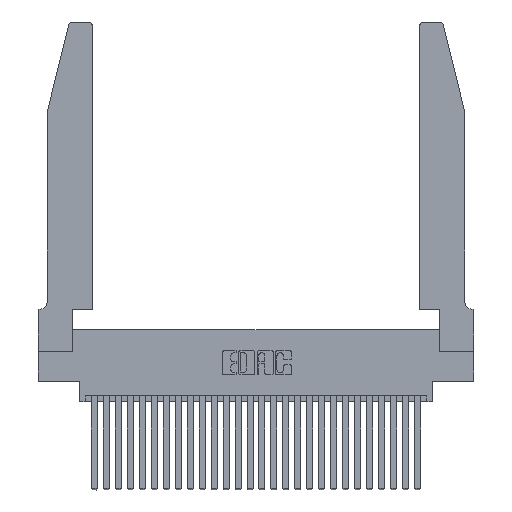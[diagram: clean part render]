
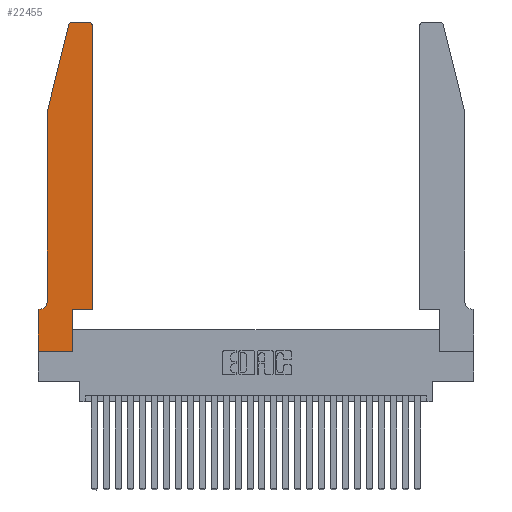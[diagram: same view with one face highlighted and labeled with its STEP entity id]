
A CAD part, top view. The second image highlights one B-rep face of the part: STEP entity #22455.
In plain terms, the highlighted planar face has unit normal (0, 0, 1).
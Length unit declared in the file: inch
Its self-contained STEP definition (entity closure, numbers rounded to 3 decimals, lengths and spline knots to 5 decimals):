
#555 = ORIENTED_EDGE ( 'NONE', *, *, #14926, .T. ) ;
#809 = LINE ( 'NONE', #10929, #18727 ) ;
#886 = VECTOR ( 'NONE', #12342, 39.37008 ) ;
#1032 = FACE_OUTER_BOUND ( 'NONE', #3108, .T. ) ;
#1141 = LINE ( 'NONE', #8079, #18023 ) ;
#1280 = CARTESIAN_POINT ( 'NONE',  ( 0.4505, 0.35, 0.37 ) ) ;
#1431 = DIRECTION ( 'NONE',  ( 0., -1., 0. ) ) ;
#1756 = CIRCLE ( 'NONE', #17456, 0.03 ) ;
#2017 = EDGE_CURVE ( 'NONE', #20932, #25572, #809, .T. ) ;
#2096 = VECTOR ( 'NONE', #15085, 39.37008 ) ;
#2839 = AXIS2_PLACEMENT_3D ( 'NONE', #10246, #25008, #14597 ) ;
#3080 = CARTESIAN_POINT ( 'NONE',  ( 0.0755, 0.42, 0.37 ) ) ;
#3108 = EDGE_LOOP ( 'NONE', ( #25094, #14569, #14059, #19852, #27587, #10947, #14539, #6120, #27247, #14308, #555, #8630 ) ) ;
#3259 = DIRECTION ( 'NONE',  ( 0., 1., 0. ) ) ;
#3295 = EDGE_CURVE ( 'NONE', #26313, #27254, #21289, .T. ) ;
#4776 = LINE ( 'NONE', #20513, #22748 ) ;
#6120 = ORIENTED_EDGE ( 'NONE', *, *, #21121, .T. ) ;
#6357 = DIRECTION ( 'NONE',  ( 0., 0., 1. ) ) ;
#6459 = DIRECTION ( 'NONE',  ( 1., 0., 0. ) ) ;
#7037 = CIRCLE ( 'NONE', #2839, 0.07 ) ;
#7141 = VECTOR ( 'NONE', #25775, 39.37008 ) ;
#7900 = CARTESIAN_POINT ( 'NONE',  ( 0., 0.35, 0.37 ) ) ;
#8079 = CARTESIAN_POINT ( 'NONE',  ( 0.2605, 2.75, 0.37 ) ) ;
#8630 = ORIENTED_EDGE ( 'NONE', *, *, #21294, .T. ) ;
#9148 = CARTESIAN_POINT ( 'NONE',  ( 0.0755, 2., 0.37 ) ) ;
#10246 = CARTESIAN_POINT ( 'NONE',  ( 0.0055, 0.42, 0.37 ) ) ;
#10405 = LINE ( 'NONE', #14263, #11792 ) ;
#10929 = CARTESIAN_POINT ( 'NONE',  ( 0.2865, 0.35, 0.37 ) ) ;
#10947 = ORIENTED_EDGE ( 'NONE', *, *, #24647, .T. ) ;
#10954 = VECTOR ( 'NONE', #1431, 39.37008 ) ;
#10977 = CIRCLE ( 'NONE', #26150, 0.03 ) ;
#11433 = VERTEX_POINT ( 'NONE', #24016 ) ;
#11792 = VECTOR ( 'NONE', #25927, 39.37008 ) ;
#12327 = EDGE_CURVE ( 'NONE', #14386, #12362, #7037, .T. ) ;
#12342 = DIRECTION ( 'NONE',  ( -1., 0., 0. ) ) ;
#12362 = VERTEX_POINT ( 'NONE', #25593 ) ;
#13050 = PLANE ( 'NONE',  #22634 ) ;
#13128 = EDGE_CURVE ( 'NONE', #15582, #18168, #1141, .T. ) ;
#13220 = DIRECTION ( 'NONE',  ( 0., 0., 1. ) ) ;
#13303 = VERTEX_POINT ( 'NONE', #15003 ) ;
#14027 = CARTESIAN_POINT ( 'NONE',  ( 0.2865, 0.35, 0.37 ) ) ;
#14059 = ORIENTED_EDGE ( 'NONE', *, *, #27819, .T. ) ;
#14208 = CARTESIAN_POINT ( 'NONE',  ( 0.284, 2.75, 0.37 ) ) ;
#14263 = CARTESIAN_POINT ( 'NONE',  ( 0., 0., 0.37 ) ) ;
#14308 = ORIENTED_EDGE ( 'NONE', *, *, #24671, .T. ) ;
#14386 = VERTEX_POINT ( 'NONE', #3080 ) ;
#14418 = CARTESIAN_POINT ( 'NONE',  ( 0.0755, 2., 0.37 ) ) ;
#14539 = ORIENTED_EDGE ( 'NONE', *, *, #3295, .T. ) ;
#14569 = ORIENTED_EDGE ( 'NONE', *, *, #23015, .T. ) ;
#14597 = DIRECTION ( 'NONE',  ( -1., 0., 0. ) ) ;
#14926 = EDGE_CURVE ( 'NONE', #11433, #27284, #4776, .T. ) ;
#14997 = VECTOR ( 'NONE', #27799, 39.37008 ) ;
#15003 = CARTESIAN_POINT ( 'NONE',  ( 0.25487, 2.72718, 0.37 ) ) ;
#15085 = DIRECTION ( 'NONE',  ( -0.239, -0.971, 0. ) ) ;
#15582 = VERTEX_POINT ( 'NONE', #20960 ) ;
#16284 = EDGE_CURVE ( 'NONE', #16912, #14386, #25075, .T. ) ;
#16912 = VERTEX_POINT ( 'NONE', #9148 ) ;
#17456 = AXIS2_PLACEMENT_3D ( 'NONE', #28552, #6357, #23908 ) ;
#17584 = CARTESIAN_POINT ( 'NONE',  ( 0., 0.35, 0.37 ) ) ;
#17900 = CARTESIAN_POINT ( 'NONE',  ( 0.4505, 2.72, 0.37 ) ) ;
#18023 = VECTOR ( 'NONE', #25754, 39.37008 ) ;
#18168 = VERTEX_POINT ( 'NONE', #14208 ) ;
#18449 = LINE ( 'NONE', #23044, #886 ) ;
#18727 = VECTOR ( 'NONE', #26169, 39.37008 ) ;
#19852 = ORIENTED_EDGE ( 'NONE', *, *, #16284, .T. ) ;
#20513 = CARTESIAN_POINT ( 'NONE',  ( 0.4505, 0.35, 0.37 ) ) ;
#20932 = VERTEX_POINT ( 'NONE', #27212 ) ;
#20960 = CARTESIAN_POINT ( 'NONE',  ( 0.4205, 2.75, 0.37 ) ) ;
#21121 = EDGE_CURVE ( 'NONE', #27254, #20932, #10405, .T. ) ;
#21289 = LINE ( 'NONE', #28011, #7141 ) ;
#21294 = EDGE_CURVE ( 'NONE', #27284, #15582, #1756, .T. ) ;
#21566 = LINE ( 'NONE', #1280, #14997 ) ;
#21748 = CARTESIAN_POINT ( 'NONE',  ( 0.0755, 2., 0.37 ) ) ;
#21924 = DIRECTION ( 'NONE',  ( 1., 0., 0. ) ) ;
#22164 = CARTESIAN_POINT ( 'NONE',  ( 0., 0., 0.37 ) ) ;
#22455 = ADVANCED_FACE ( 'NONE', ( #1032 ), #13050, .T. ) ;
#22634 = AXIS2_PLACEMENT_3D ( 'NONE', #17584, #28494, #21924 ) ;
#22748 = VECTOR ( 'NONE', #3259, 39.37008 ) ;
#23015 = EDGE_CURVE ( 'NONE', #18168, #13303, #10977, .T. ) ;
#23044 = CARTESIAN_POINT ( 'NONE',  ( 0.0755, 0.35, 0.37 ) ) ;
#23908 = DIRECTION ( 'NONE',  ( 1., 0., 0. ) ) ;
#24016 = CARTESIAN_POINT ( 'NONE',  ( 0.4505, 0.35, 0.37 ) ) ;
#24219 = CARTESIAN_POINT ( 'NONE',  ( 0.284, 2.72, 0.37 ) ) ;
#24647 = EDGE_CURVE ( 'NONE', #12362, #26313, #18449, .T. ) ;
#24671 = EDGE_CURVE ( 'NONE', #25572, #11433, #21566, .T. ) ;
#25008 = DIRECTION ( 'NONE',  ( 0., 0., -1. ) ) ;
#25075 = LINE ( 'NONE', #14418, #10954 ) ;
#25094 = ORIENTED_EDGE ( 'NONE', *, *, #13128, .T. ) ;
#25572 = VERTEX_POINT ( 'NONE', #14027 ) ;
#25593 = CARTESIAN_POINT ( 'NONE',  ( 0.0055, 0.35, 0.37 ) ) ;
#25754 = DIRECTION ( 'NONE',  ( -1., 0., 0. ) ) ;
#25775 = DIRECTION ( 'NONE',  ( 0., -1., 0. ) ) ;
#25927 = DIRECTION ( 'NONE',  ( 1., 0., 0. ) ) ;
#26150 = AXIS2_PLACEMENT_3D ( 'NONE', #24219, #13220, #6459 ) ;
#26169 = DIRECTION ( 'NONE',  ( 0., 1., 0. ) ) ;
#26313 = VERTEX_POINT ( 'NONE', #7900 ) ;
#27212 = CARTESIAN_POINT ( 'NONE',  ( 0.2865, 0., 0.37 ) ) ;
#27247 = ORIENTED_EDGE ( 'NONE', *, *, #2017, .T. ) ;
#27254 = VERTEX_POINT ( 'NONE', #22164 ) ;
#27284 = VERTEX_POINT ( 'NONE', #17900 ) ;
#27587 = ORIENTED_EDGE ( 'NONE', *, *, #12327, .T. ) ;
#27639 = LINE ( 'NONE', #21748, #2096 ) ;
#27799 = DIRECTION ( 'NONE',  ( 1., 0., 0. ) ) ;
#27819 = EDGE_CURVE ( 'NONE', #13303, #16912, #27639, .T. ) ;
#28011 = CARTESIAN_POINT ( 'NONE',  ( 0., 0., 0.37 ) ) ;
#28494 = DIRECTION ( 'NONE',  ( 0., 0., 1. ) ) ;
#28552 = CARTESIAN_POINT ( 'NONE',  ( 0.4205, 2.72, 0.37 ) ) ;
